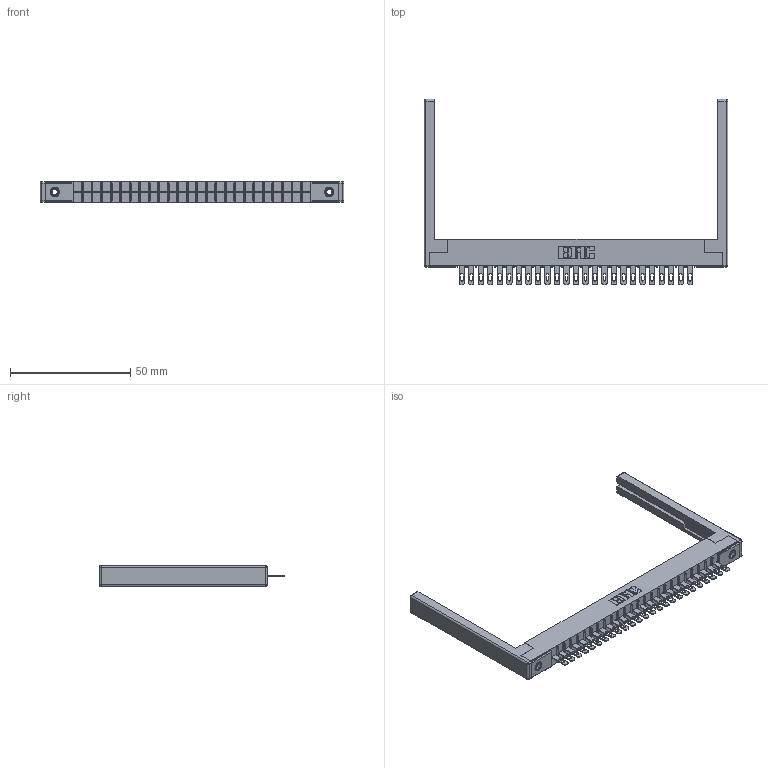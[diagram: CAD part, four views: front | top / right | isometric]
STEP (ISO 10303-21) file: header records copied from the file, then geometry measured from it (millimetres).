
FILE_DESCRIPTION (( 'STEP AP203' ), '1' );
FILE_NAME ('356-025-500-168.STEP', '2018-08-01T20:14:56', ( '' ), ( '' ), 'SwSTEP 2.0', 'SolidWorks 2016', '' );
FILE_SCHEMA (( 'CONFIG_CONTROL_DESIGN' ));
Length unit declared in the file: inch
Products named in the file (5): 306 Part_.156 Dia; 306-290-001_100; 345-250-001_345-250-001-102; 307-220-068; 356-025-500-168
Assembly tree (30 placements, depth 2):
  356-025-500-168
    306 Part_.156 Dia
    306-290-001_100  x25
    345-250-001_345-250-001-102  x2
    307-220-068  x2
Bounding box: 126.49 x 77.17 x 8.71 mm (x, y, z)
Volume: 13289 mm3; surface area: 17537.4 mm2
Topology: 30 solids, 30 shells, 2170 faces, 6081 edges, 3898 vertices
Faces by surface type: plane 1406, cylinder 640, sphere 108, cone 12, torus 4
Entity records: 28439 total; most frequent: CARTESIAN_POINT 4739, ORIENTED_EDGE 4688, DIRECTION 4688, EDGE_CURVE 2344, VECTOR 1818, LINE 1818, VERTEX_POINT 1486, AXIS2_PLACEMENT_3D 1435
